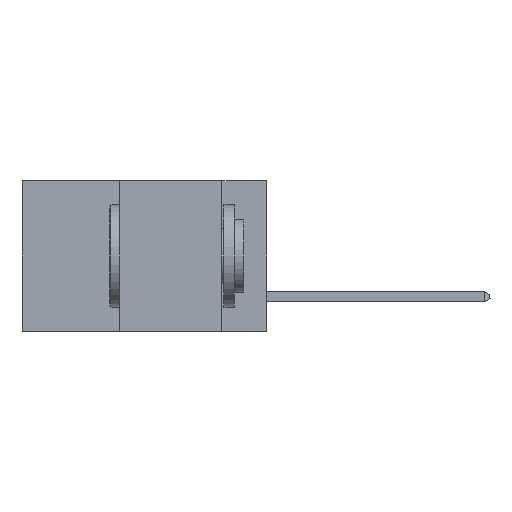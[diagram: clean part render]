
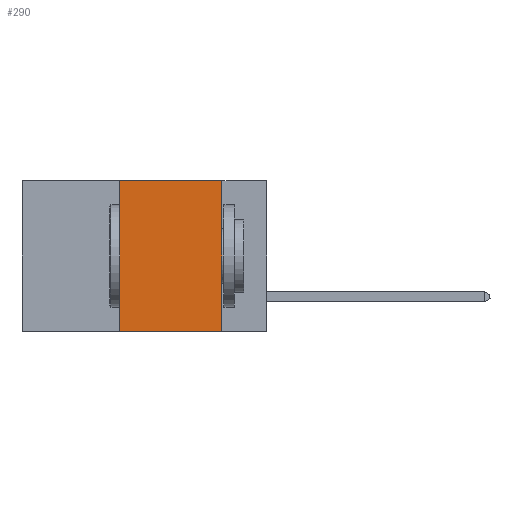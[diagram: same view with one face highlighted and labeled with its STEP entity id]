
A CAD part, left-side view. The second image highlights one B-rep face of the part: STEP entity #290.
In plain terms, the highlighted planar face has unit normal (-1, 0, 0).
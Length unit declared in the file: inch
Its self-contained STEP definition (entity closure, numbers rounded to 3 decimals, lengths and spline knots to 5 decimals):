
#290 = ADVANCED_FACE ( 'NONE', ( #3604 ), #9190, .F. ) ;
#658 = LINE ( 'NONE', #7741, #1203 ) ;
#1129 = LINE ( 'NONE', #10006, #2457 ) ;
#1203 = VECTOR ( 'NONE', #9623, 39.37008 ) ;
#1292 = VECTOR ( 'NONE', #11433, 39.37008 ) ;
#1894 = DIRECTION ( 'NONE',  ( 0., 0., 1. ) ) ;
#1972 = EDGE_CURVE ( 'NONE', #7598, #3856, #9517, .T. ) ;
#2457 = VECTOR ( 'NONE', #1894, 39.37008 ) ;
#2621 = VERTEX_POINT ( 'NONE', #5054 ) ;
#2853 = ORIENTED_EDGE ( 'NONE', *, *, #9136, .F. ) ;
#2930 = EDGE_CURVE ( 'NONE', #2621, #3856, #658, .T. ) ;
#3604 = FACE_OUTER_BOUND ( 'NONE', #4279, .T. ) ;
#3801 = VERTEX_POINT ( 'NONE', #10083 ) ;
#3856 = VERTEX_POINT ( 'NONE', #11501 ) ;
#4279 = EDGE_LOOP ( 'NONE', ( #7413, #2853, #6860, #9801 ) ) ;
#4526 = DIRECTION ( 'NONE',  ( 0., 0., -1. ) ) ;
#4602 = DIRECTION ( 'NONE',  ( 1., 0., 0. ) ) ;
#5054 = CARTESIAN_POINT ( 'NONE',  ( 0., 0.36, -0.37 ) ) ;
#5419 = CARTESIAN_POINT ( 'NONE',  ( 0., 0.11, 0. ) ) ;
#5612 = EDGE_CURVE ( 'NONE', #2621, #3801, #1129, .T. ) ;
#6101 = LINE ( 'NONE', #7574, #1292 ) ;
#6860 = ORIENTED_EDGE ( 'NONE', *, *, #5612, .F. ) ;
#7268 = DIRECTION ( 'NONE',  ( 0., 0., -1. ) ) ;
#7413 = ORIENTED_EDGE ( 'NONE', *, *, #1972, .F. ) ;
#7574 = CARTESIAN_POINT ( 'NONE',  ( 0., 0.6, 0. ) ) ;
#7598 = VERTEX_POINT ( 'NONE', #11595 ) ;
#7741 = CARTESIAN_POINT ( 'NONE',  ( 0., 0.6, -0.37 ) ) ;
#9136 = EDGE_CURVE ( 'NONE', #3801, #7598, #6101, .T. ) ;
#9190 = PLANE ( 'NONE',  #10839 ) ;
#9246 = VECTOR ( 'NONE', #7268, 39.37008 ) ;
#9517 = LINE ( 'NONE', #5419, #9246 ) ;
#9623 = DIRECTION ( 'NONE',  ( 0., -1., 0. ) ) ;
#9801 = ORIENTED_EDGE ( 'NONE', *, *, #2930, .T. ) ;
#10006 = CARTESIAN_POINT ( 'NONE',  ( 0., 0.36, 0. ) ) ;
#10083 = CARTESIAN_POINT ( 'NONE',  ( 0., 0.36, 0. ) ) ;
#10839 = AXIS2_PLACEMENT_3D ( 'NONE', #10986, #4602, #4526 ) ;
#10986 = CARTESIAN_POINT ( 'NONE',  ( 0., 0.6, 0. ) ) ;
#11433 = DIRECTION ( 'NONE',  ( 0., -1., 0. ) ) ;
#11501 = CARTESIAN_POINT ( 'NONE',  ( 0., 0.11, -0.37 ) ) ;
#11595 = CARTESIAN_POINT ( 'NONE',  ( 0., 0.11, 0. ) ) ;
